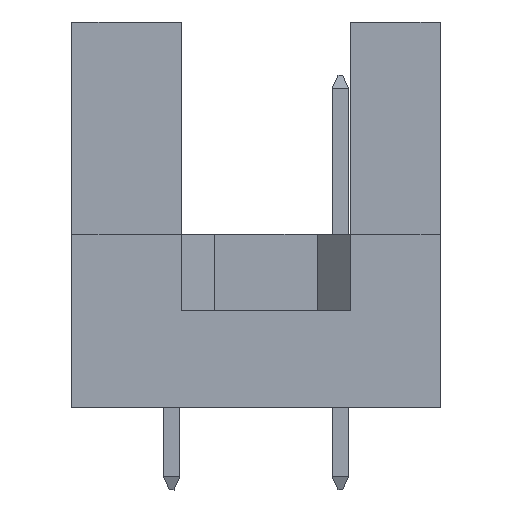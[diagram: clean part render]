
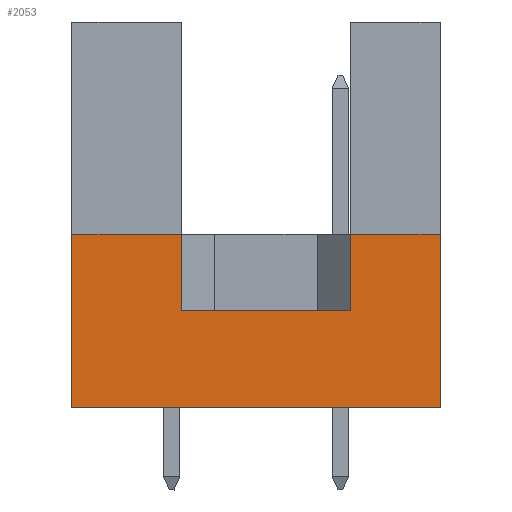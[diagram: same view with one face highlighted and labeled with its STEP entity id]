
A CAD part, left-side view. The second image highlights one B-rep face of the part: STEP entity #2053.
In plain terms, the highlighted planar face has unit normal (-1, 0, 0).
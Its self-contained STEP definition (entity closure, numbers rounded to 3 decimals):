
#326 = ORIENTED_EDGE ( 'NONE', *, *, #4607, .F. ) ;
#330 = EDGE_CURVE ( 'NONE', #8058, #8730, #6381, .T. ) ;
#445 = CARTESIAN_POINT ( 'NONE',  ( -27.5, 11.1, 0. ) ) ;
#523 = CARTESIAN_POINT ( 'NONE',  ( -27.5, 0., 0. ) ) ;
#586 = CARTESIAN_POINT ( 'NONE',  ( -27.5, 2.71, 5.2 ) ) ;
#717 = CARTESIAN_POINT ( 'NONE',  ( -27.5, 0., 5.2 ) ) ;
#812 = VERTEX_POINT ( 'NONE', #717 ) ;
#851 = ORIENTED_EDGE ( 'NONE', *, *, #6009, .F. ) ;
#1082 = CARTESIAN_POINT ( 'NONE',  ( -27.5, 11.1, 5.2 ) ) ;
#1100 = LINE ( 'NONE', #445, #5505 ) ;
#1152 = PLANE ( 'NONE',  #8347 ) ;
#1200 = VERTEX_POINT ( 'NONE', #5221 ) ;
#1365 = ORIENTED_EDGE ( 'NONE', *, *, #8508, .T. ) ;
#1487 = ORIENTED_EDGE ( 'NONE', *, *, #3382, .F. ) ;
#1737 = CARTESIAN_POINT ( 'NONE',  ( -27.5, 7.79, 5.2 ) ) ;
#2053 = ADVANCED_FACE ( 'NONE', ( #8776 ), #1152, .F. ) ;
#2299 = LINE ( 'NONE', #5352, #2471 ) ;
#2366 = LINE ( 'NONE', #4574, #9314 ) ;
#2433 = VECTOR ( 'NONE', #5876, 1000. ) ;
#2471 = VECTOR ( 'NONE', #8383, 1000. ) ;
#2536 = CARTESIAN_POINT ( 'NONE',  ( -27.5, 7.79, 2.9 ) ) ;
#2783 = LINE ( 'NONE', #3996, #8254 ) ;
#3022 = ORIENTED_EDGE ( 'NONE', *, *, #9299, .F. ) ;
#3200 = CARTESIAN_POINT ( 'NONE',  ( -27.5, 11.1, 0. ) ) ;
#3382 = EDGE_CURVE ( 'NONE', #6814, #4669, #2299, .T. ) ;
#3414 = ORIENTED_EDGE ( 'NONE', *, *, #330, .T. ) ;
#3528 = EDGE_CURVE ( 'NONE', #4566, #1200, #1100, .T. ) ;
#3530 = VERTEX_POINT ( 'NONE', #9673 ) ;
#3543 = CARTESIAN_POINT ( 'NONE',  ( -27.5, 7.79, 2.9 ) ) ;
#3966 = DIRECTION ( 'NONE',  ( 0., -1., 0. ) ) ;
#3996 = CARTESIAN_POINT ( 'NONE',  ( -27.5, 11.1, 0. ) ) ;
#4052 = EDGE_LOOP ( 'NONE', ( #851, #3414, #4573, #326, #8106, #1365, #3022, #1487 ) ) ;
#4122 = DIRECTION ( 'NONE',  ( 0., -1., 0. ) ) ;
#4312 = VECTOR ( 'NONE', #6342, 1000. ) ;
#4566 = VERTEX_POINT ( 'NONE', #3200 ) ;
#4573 = ORIENTED_EDGE ( 'NONE', *, *, #5336, .F. ) ;
#4574 = CARTESIAN_POINT ( 'NONE',  ( -27.5, 11.1, 5.2 ) ) ;
#4607 = EDGE_CURVE ( 'NONE', #4566, #3530, #2783, .T. ) ;
#4669 = VERTEX_POINT ( 'NONE', #586 ) ;
#4721 = CARTESIAN_POINT ( 'NONE',  ( -27.5, 2.71, 2.9 ) ) ;
#5221 = CARTESIAN_POINT ( 'NONE',  ( -27.5, 0., 0. ) ) ;
#5336 = EDGE_CURVE ( 'NONE', #3530, #8730, #2366, .T. ) ;
#5352 = CARTESIAN_POINT ( 'NONE',  ( -27.5, 2.71, 2.9 ) ) ;
#5505 = VECTOR ( 'NONE', #7270, 1000. ) ;
#5593 = LINE ( 'NONE', #9423, #4312 ) ;
#5620 = LINE ( 'NONE', #1082, #8981 ) ;
#5876 = DIRECTION ( 'NONE',  ( 0., 0., 1. ) ) ;
#6009 = EDGE_CURVE ( 'NONE', #8058, #6814, #5593, .T. ) ;
#6342 = DIRECTION ( 'NONE',  ( 0., -1., 0. ) ) ;
#6381 = LINE ( 'NONE', #2536, #8086 ) ;
#6467 = LINE ( 'NONE', #523, #2433 ) ;
#6531 = DIRECTION ( 'NONE',  ( 1., 0., 0. ) ) ;
#6631 = CARTESIAN_POINT ( 'NONE',  ( -27.5, 11.1, 0. ) ) ;
#6814 = VERTEX_POINT ( 'NONE', #4721 ) ;
#7261 = DIRECTION ( 'NONE',  ( 0., 0., 1. ) ) ;
#7270 = DIRECTION ( 'NONE',  ( 0., -1., 0. ) ) ;
#8058 = VERTEX_POINT ( 'NONE', #3543 ) ;
#8086 = VECTOR ( 'NONE', #8574, 1000. ) ;
#8106 = ORIENTED_EDGE ( 'NONE', *, *, #3528, .T. ) ;
#8254 = VECTOR ( 'NONE', #7261, 1000. ) ;
#8347 = AXIS2_PLACEMENT_3D ( 'NONE', #6631, #6531, #9471 ) ;
#8383 = DIRECTION ( 'NONE',  ( 0., 0., 1. ) ) ;
#8508 = EDGE_CURVE ( 'NONE', #1200, #812, #6467, .T. ) ;
#8574 = DIRECTION ( 'NONE',  ( 0., 0., 1. ) ) ;
#8730 = VERTEX_POINT ( 'NONE', #1737 ) ;
#8776 = FACE_OUTER_BOUND ( 'NONE', #4052, .T. ) ;
#8981 = VECTOR ( 'NONE', #4122, 1000. ) ;
#9299 = EDGE_CURVE ( 'NONE', #4669, #812, #5620, .T. ) ;
#9314 = VECTOR ( 'NONE', #3966, 1000. ) ;
#9423 = CARTESIAN_POINT ( 'NONE',  ( -27.5, 7.79, 2.9 ) ) ;
#9471 = DIRECTION ( 'NONE',  ( 0., 0., -1. ) ) ;
#9673 = CARTESIAN_POINT ( 'NONE',  ( -27.5, 11.1, 5.2 ) ) ;
